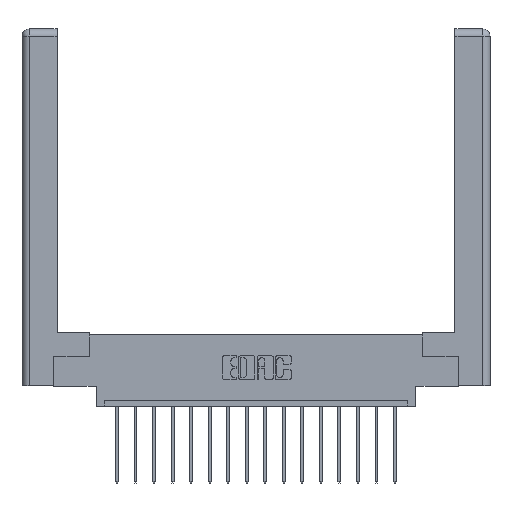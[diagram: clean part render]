
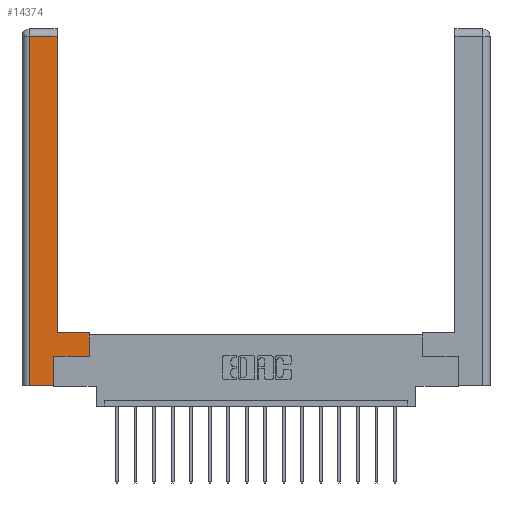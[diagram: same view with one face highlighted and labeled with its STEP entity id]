
A CAD part, top view. The second image highlights one B-rep face of the part: STEP entity #14374.
In plain terms, the highlighted planar face has unit normal (0, 0, 1).
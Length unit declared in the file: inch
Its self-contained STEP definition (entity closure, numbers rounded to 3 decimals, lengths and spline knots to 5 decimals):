
#21 = CARTESIAN_POINT ( 'NONE',  ( 0.0615, 2.94, 0. ) ) ;
#287 = DIRECTION ( 'NONE',  ( 1., 0., 0. ) ) ;
#441 = ORIENTED_EDGE ( 'NONE', *, *, #16826, .T. ) ;
#554 = EDGE_CURVE ( 'NONE', #2198, #16562, #2664, .T. ) ;
#966 = DIRECTION ( 'NONE',  ( 0., -1., 0. ) ) ;
#1105 = CARTESIAN_POINT ( 'NONE',  ( 0.565, 0.45, 0. ) ) ;
#1156 = DIRECTION ( 'NONE',  ( -1., 0., 0. ) ) ;
#1645 = VERTEX_POINT ( 'NONE', #15588 ) ;
#1687 = ORIENTED_EDGE ( 'NONE', *, *, #16224, .T. ) ;
#1731 = DIRECTION ( 'NONE',  ( 0., 0., -1. ) ) ;
#1761 = CARTESIAN_POINT ( 'NONE',  ( 0.565, 0.45, 0. ) ) ;
#2117 = CARTESIAN_POINT ( 'NONE',  ( 0.265, 0.245, 0. ) ) ;
#2198 = VERTEX_POINT ( 'NONE', #8563 ) ;
#2653 = LINE ( 'NONE', #15232, #13115 ) ;
#2664 = LINE ( 'NONE', #2117, #5276 ) ;
#3134 = FACE_OUTER_BOUND ( 'NONE', #14421, .T. ) ;
#3291 = CARTESIAN_POINT ( 'NONE',  ( 0., 0., 0. ) ) ;
#3320 = LINE ( 'NONE', #21, #3523 ) ;
#3523 = VECTOR ( 'NONE', #1156, 39.37008 ) ;
#3727 = DIRECTION ( 'NONE',  ( 0., 1., 0. ) ) ;
#3961 = ORIENTED_EDGE ( 'NONE', *, *, #4744, .T. ) ;
#4744 = EDGE_CURVE ( 'NONE', #17541, #10892, #8113, .T. ) ;
#4891 = CARTESIAN_POINT ( 'NONE',  ( 0.0615, 0., 0. ) ) ;
#5070 = CARTESIAN_POINT ( 'NONE',  ( 0.295, 0.45, 0. ) ) ;
#5276 = VECTOR ( 'NONE', #16129, 39.37008 ) ;
#5545 = LINE ( 'NONE', #7228, #14472 ) ;
#5594 = EDGE_CURVE ( 'NONE', #16562, #17541, #2653, .T. ) ;
#6456 = ORIENTED_EDGE ( 'NONE', *, *, #5594, .T. ) ;
#6796 = AXIS2_PLACEMENT_3D ( 'NONE', #3291, #1731, #11473 ) ;
#7009 = LINE ( 'NONE', #4891, #7460 ) ;
#7183 = VECTOR ( 'NONE', #8398, 39.37008 ) ;
#7228 = CARTESIAN_POINT ( 'NONE',  ( 0.265, 0., 0. ) ) ;
#7271 = PLANE ( 'NONE',  #6796 ) ;
#7460 = VECTOR ( 'NONE', #966, 39.37008 ) ;
#7500 = VERTEX_POINT ( 'NONE', #8060 ) ;
#7839 = ORIENTED_EDGE ( 'NONE', *, *, #554, .T. ) ;
#8060 = CARTESIAN_POINT ( 'NONE',  ( 0.0615, 0., 0. ) ) ;
#8113 = LINE ( 'NONE', #1761, #15766 ) ;
#8147 = CARTESIAN_POINT ( 'NONE',  ( 0.565, 0.245, 0. ) ) ;
#8272 = CARTESIAN_POINT ( 'NONE',  ( 0.295, 0.45, 0. ) ) ;
#8398 = DIRECTION ( 'NONE',  ( -1., 0., 0. ) ) ;
#8470 = EDGE_CURVE ( 'NONE', #13969, #1645, #3320, .T. ) ;
#8563 = CARTESIAN_POINT ( 'NONE',  ( 0.265, 0., 0. ) ) ;
#9126 = ORIENTED_EDGE ( 'NONE', *, *, #13691, .T. ) ;
#10006 = EDGE_CURVE ( 'NONE', #15315, #13969, #16493, .T. ) ;
#10129 = CARTESIAN_POINT ( 'NONE',  ( 0.265, 0.245, 0. ) ) ;
#10881 = LINE ( 'NONE', #8272, #7183 ) ;
#10892 = VERTEX_POINT ( 'NONE', #1105 ) ;
#11473 = DIRECTION ( 'NONE',  ( -1., 0., 0. ) ) ;
#11885 = CARTESIAN_POINT ( 'NONE',  ( 0.295, 2.94, 0. ) ) ;
#12299 = DIRECTION ( 'NONE',  ( 1., 0., 0. ) ) ;
#12315 = CARTESIAN_POINT ( 'NONE',  ( 0.295, 3., 0. ) ) ;
#13115 = VECTOR ( 'NONE', #12299, 39.37008 ) ;
#13691 = EDGE_CURVE ( 'NONE', #7500, #2198, #5545, .T. ) ;
#13969 = VERTEX_POINT ( 'NONE', #11885 ) ;
#14374 = ADVANCED_FACE ( 'NONE', ( #3134 ), #7271, .F. ) ;
#14421 = EDGE_LOOP ( 'NONE', ( #18067, #15205, #441, #9126, #7839, #6456, #3961, #1687 ) ) ;
#14472 = VECTOR ( 'NONE', #287, 39.37008 ) ;
#15003 = DIRECTION ( 'NONE',  ( 0., 1., 0. ) ) ;
#15205 = ORIENTED_EDGE ( 'NONE', *, *, #8470, .T. ) ;
#15232 = CARTESIAN_POINT ( 'NONE',  ( 0.565, 0.245, 0. ) ) ;
#15315 = VERTEX_POINT ( 'NONE', #5070 ) ;
#15588 = CARTESIAN_POINT ( 'NONE',  ( 0.0615, 2.94, 0. ) ) ;
#15766 = VECTOR ( 'NONE', #3727, 39.37008 ) ;
#16129 = DIRECTION ( 'NONE',  ( 0., 1., 0. ) ) ;
#16224 = EDGE_CURVE ( 'NONE', #10892, #15315, #10881, .T. ) ;
#16493 = LINE ( 'NONE', #12315, #16723 ) ;
#16562 = VERTEX_POINT ( 'NONE', #10129 ) ;
#16723 = VECTOR ( 'NONE', #15003, 39.37008 ) ;
#16826 = EDGE_CURVE ( 'NONE', #1645, #7500, #7009, .T. ) ;
#17541 = VERTEX_POINT ( 'NONE', #8147 ) ;
#18067 = ORIENTED_EDGE ( 'NONE', *, *, #10006, .T. ) ;
